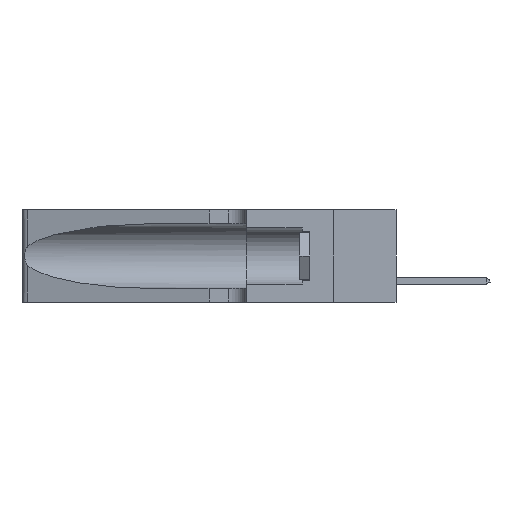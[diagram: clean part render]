
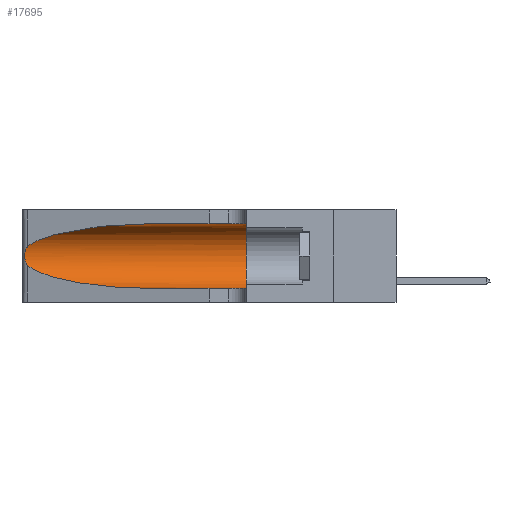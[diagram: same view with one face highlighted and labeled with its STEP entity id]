
A CAD part, left-side view. The second image highlights one B-rep face of the part: STEP entity #17695.
In plain terms, the highlighted cylindrical face has radius 3.308 mm (diameter 6.617 mm), a partial arc.
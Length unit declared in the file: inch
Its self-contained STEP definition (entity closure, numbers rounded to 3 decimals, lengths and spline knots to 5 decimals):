
#708 = EDGE_CURVE ( 'NONE', #26337, #983, #22146, .T. ) ;
#801 =( BOUNDED_CURVE ( )  B_SPLINE_CURVE ( 3, ( #11208, #3725, #8917, #31517 ),
 .UNSPECIFIED., .F., .F. ) 
 B_SPLINE_CURVE_WITH_KNOTS ( ( 4, 4 ),
 ( 1.5708, 2.84003 ),
 .UNSPECIFIED. ) 
 CURVE ( )  GEOMETRIC_REPRESENTATION_ITEM ( )  RATIONAL_B_SPLINE_CURVE ( ( 1., 0.87, 0.87, 1. ) ) 
 REPRESENTATION_ITEM ( '' )  );
#983 = VERTEX_POINT ( 'NONE', #2152 ) ;
#991 = VERTEX_POINT ( 'NONE', #7646 ) ;
#1512 = EDGE_LOOP ( 'NONE', ( #5094, #7626, #4486, #28306, #10178, #7216 ) ) ;
#1556 = CARTESIAN_POINT ( 'NONE',  ( 0.26075, 1.23896, 0.178 ) ) ;
#2083 = VECTOR ( 'NONE', #26777, 39.37008 ) ;
#2084 = CARTESIAN_POINT ( 'NONE',  ( 0.25487, 1.22718, 0.14631 ) ) ;
#2142 = CIRCLE ( 'NONE', #11233, 0.13025 ) ;
#2152 = CARTESIAN_POINT ( 'NONE',  ( 0.1305, 0.35, 0.31525 ) ) ;
#2782 = B_SPLINE_CURVE_WITH_KNOTS ( 'NONE', 3,
 ( #26630, #19365, #16931, #27060, #9058, #9153, #16498, #1556, #14547, #26945, #19036, #21894, #24432, #14449 ),
 .UNSPECIFIED., .F., .F.,
 ( 4, 2, 2, 2, 2, 2, 4 ),
 ( 0., 0.00027, 0.00053, 0.00107, 0.0016, 0.00187, 0.00214 ),
 .UNSPECIFIED. ) ;
#3725 = CARTESIAN_POINT ( 'NONE',  ( 0.18966, 0.96281, 0.31525 ) ) ;
#4429 = DIRECTION ( 'NONE',  ( 0., 0., 1. ) ) ;
#4486 = ORIENTED_EDGE ( 'NONE', *, *, #30706, .T. ) ;
#5094 = ORIENTED_EDGE ( 'NONE', *, *, #23006, .T. ) ;
#6698 = DIRECTION ( 'NONE',  ( 0., -1., 0. ) ) ;
#6750 = CARTESIAN_POINT ( 'NONE',  ( 0.1305, 0.35, 0.185 ) ) ;
#7180 = CARTESIAN_POINT ( 'NONE',  ( 0.1305, 0.72297, 0.05475 ) ) ;
#7216 = ORIENTED_EDGE ( 'NONE', *, *, #708, .F. ) ;
#7626 = ORIENTED_EDGE ( 'NONE', *, *, #32434, .T. ) ;
#7646 = CARTESIAN_POINT ( 'NONE',  ( 0.1305, 0.72297, 0.05475 ) ) ;
#8917 = CARTESIAN_POINT ( 'NONE',  ( 0.2373, 1.15595, 0.28018 ) ) ;
#9058 = CARTESIAN_POINT ( 'NONE',  ( 0.25854, 1.2359, 0.20912 ) ) ;
#9153 = CARTESIAN_POINT ( 'NONE',  ( 0.26018, 1.23835, 0.19895 ) ) ;
#9291 = FACE_OUTER_BOUND ( 'NONE', #1512, .T. ) ;
#10178 = ORIENTED_EDGE ( 'NONE', *, *, #30665, .F. ) ;
#10557 = DIRECTION ( 'NONE',  ( 0., -1., 0. ) ) ;
#11208 = CARTESIAN_POINT ( 'NONE',  ( 0.1305, 0.72297, 0.31525 ) ) ;
#11233 = AXIS2_PLACEMENT_3D ( 'NONE', #6750, #24526, #4429 ) ;
#12433 = CYLINDRICAL_SURFACE ( 'NONE', #26062, 0.13025 ) ;
#13114 = CARTESIAN_POINT ( 'NONE',  ( 0.25487, 1.22718, 0.14631 ) ) ;
#13518 = VERTEX_POINT ( 'NONE', #13845 ) ;
#13845 = CARTESIAN_POINT ( 'NONE',  ( 0.1305, 0.35, 0.05475 ) ) ;
#14278 = DIRECTION ( 'NONE',  ( 0., 0., -1. ) ) ;
#14449 = CARTESIAN_POINT ( 'NONE',  ( 0.25487, 1.22718, 0.14631 ) ) ;
#14547 = CARTESIAN_POINT ( 'NONE',  ( 0.26017, 1.23833, 0.17102 ) ) ;
#16498 = CARTESIAN_POINT ( 'NONE',  ( 0.26075, 1.23896, 0.19203 ) ) ;
#16931 = CARTESIAN_POINT ( 'NONE',  ( 0.25639, 1.23184, 0.21858 ) ) ;
#17695 = ADVANCED_FACE ( 'NONE', ( #9291 ), #12433, .F. ) ;
#18623 = EDGE_CURVE ( 'NONE', #991, #13518, #28887, .T. ) ;
#19036 = CARTESIAN_POINT ( 'NONE',  ( 0.25789, 1.23486, 0.15765 ) ) ;
#19365 = CARTESIAN_POINT ( 'NONE',  ( 0.25555, 1.22994, 0.2215 ) ) ;
#19685 = CARTESIAN_POINT ( 'NONE',  ( 0.2373, 1.15595, 0.08982 ) ) ;
#21527 = VERTEX_POINT ( 'NONE', #24041 ) ;
#21888 = CARTESIAN_POINT ( 'NONE',  ( 0.18966, 0.96281, 0.05475 ) ) ;
#21894 = CARTESIAN_POINT ( 'NONE',  ( 0.25639, 1.23186, 0.15144 ) ) ;
#21940 = CARTESIAN_POINT ( 'NONE',  ( 0.1305, 1.61858, 0.31525 ) ) ;
#22146 = LINE ( 'NONE', #21940, #2083 ) ;
#22271 = VERTEX_POINT ( 'NONE', #13114 ) ;
#23006 = EDGE_CURVE ( 'NONE', #26337, #21527, #801, .T. ) ;
#24041 = CARTESIAN_POINT ( 'NONE',  ( 0.25487, 1.22718, 0.22369 ) ) ;
#24432 = CARTESIAN_POINT ( 'NONE',  ( 0.25555, 1.22993, 0.14849 ) ) ;
#24526 = DIRECTION ( 'NONE',  ( 0., 1., 0. ) ) ;
#25184 =( BOUNDED_CURVE ( )  B_SPLINE_CURVE ( 3, ( #2084, #19685, #21888, #7180 ),
 .UNSPECIFIED., .F., .F. ) 
 B_SPLINE_CURVE_WITH_KNOTS ( ( 4, 4 ),
 ( 3.44316, 4.71239 ),
 .UNSPECIFIED. ) 
 CURVE ( )  GEOMETRIC_REPRESENTATION_ITEM ( )  RATIONAL_B_SPLINE_CURVE ( ( 1., 0.87, 0.87, 1. ) ) 
 REPRESENTATION_ITEM ( '' )  );
#26062 = AXIS2_PLACEMENT_3D ( 'NONE', #27000, #6698, #14278 ) ;
#26337 = VERTEX_POINT ( 'NONE', #27476 ) ;
#26630 = CARTESIAN_POINT ( 'NONE',  ( 0.25487, 1.22718, 0.22369 ) ) ;
#26777 = DIRECTION ( 'NONE',  ( 0., -1., 0. ) ) ;
#26945 = CARTESIAN_POINT ( 'NONE',  ( 0.25856, 1.23593, 0.16098 ) ) ;
#27000 = CARTESIAN_POINT ( 'NONE',  ( 0.1305, 1.61858, 0.185 ) ) ;
#27060 = CARTESIAN_POINT ( 'NONE',  ( 0.25787, 1.23484, 0.2124 ) ) ;
#27476 = CARTESIAN_POINT ( 'NONE',  ( 0.1305, 0.72297, 0.31525 ) ) ;
#28306 = ORIENTED_EDGE ( 'NONE', *, *, #18623, .T. ) ;
#28887 = LINE ( 'NONE', #30668, #31997 ) ;
#30665 = EDGE_CURVE ( 'NONE', #983, #13518, #2142, .T. ) ;
#30668 = CARTESIAN_POINT ( 'NONE',  ( 0.1305, 1.61858, 0.05475 ) ) ;
#30706 = EDGE_CURVE ( 'NONE', #22271, #991, #25184, .T. ) ;
#31517 = CARTESIAN_POINT ( 'NONE',  ( 0.25487, 1.22718, 0.22369 ) ) ;
#31997 = VECTOR ( 'NONE', #10557, 39.37008 ) ;
#32434 = EDGE_CURVE ( 'NONE', #21527, #22271, #2782, .T. ) ;
